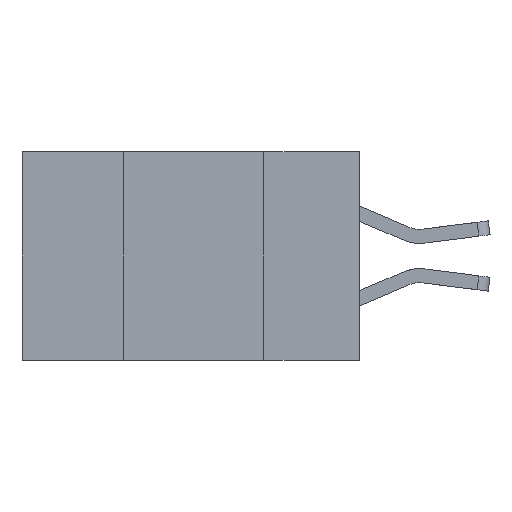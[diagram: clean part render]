
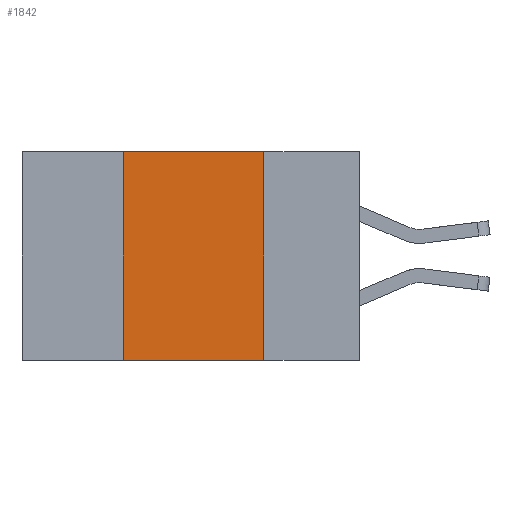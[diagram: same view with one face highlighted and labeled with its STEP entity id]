
A CAD part, left-side view. The second image highlights one B-rep face of the part: STEP entity #1842.
In plain terms, the highlighted planar face has unit normal (-1, 0, 0).
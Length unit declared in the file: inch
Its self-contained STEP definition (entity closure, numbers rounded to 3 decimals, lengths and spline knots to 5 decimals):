
#111 = FACE_OUTER_BOUND ( 'NONE', #4299, .T. ) ;
#204 = LINE ( 'NONE', #1067, #6539 ) ;
#880 = EDGE_CURVE ( 'NONE', #5905, #8308, #2870, .T. ) ;
#1003 = EDGE_CURVE ( 'NONE', #5375, #8308, #4313, .T. ) ;
#1067 = CARTESIAN_POINT ( 'NONE',  ( 0., 0.6, 0. ) ) ;
#1464 = AXIS2_PLACEMENT_3D ( 'NONE', #8762, #1615, #1802 ) ;
#1575 = VECTOR ( 'NONE', #8467, 39.37008 ) ;
#1615 = DIRECTION ( 'NONE',  ( 1., 0., 0. ) ) ;
#1802 = DIRECTION ( 'NONE',  ( 0., 0., -1. ) ) ;
#1842 = ADVANCED_FACE ( 'NONE', ( #111 ), #4460, .F. ) ;
#2870 = LINE ( 'NONE', #7503, #6959 ) ;
#2989 = CARTESIAN_POINT ( 'NONE',  ( 0., 0.42, 0. ) ) ;
#3553 = ORIENTED_EDGE ( 'NONE', *, *, #4129, .F. ) ;
#4002 = CARTESIAN_POINT ( 'NONE',  ( 0., 0.42, -0.37 ) ) ;
#4129 = EDGE_CURVE ( 'NONE', #5905, #6833, #8019, .T. ) ;
#4299 = EDGE_LOOP ( 'NONE', ( #8887, #4461, #3553, #9949 ) ) ;
#4313 = LINE ( 'NONE', #8397, #1575 ) ;
#4460 = PLANE ( 'NONE',  #1464 ) ;
#4461 = ORIENTED_EDGE ( 'NONE', *, *, #9060, .F. ) ;
#5375 = VERTEX_POINT ( 'NONE', #10539 ) ;
#5905 = VERTEX_POINT ( 'NONE', #4002 ) ;
#6155 = VECTOR ( 'NONE', #7654, 39.37008 ) ;
#6539 = VECTOR ( 'NONE', #10090, 39.37008 ) ;
#6833 = VERTEX_POINT ( 'NONE', #2989 ) ;
#6959 = VECTOR ( 'NONE', #9754, 39.37008 ) ;
#7503 = CARTESIAN_POINT ( 'NONE',  ( 0., 0.6, -0.37 ) ) ;
#7654 = DIRECTION ( 'NONE',  ( 0., 0., 1. ) ) ;
#7668 = CARTESIAN_POINT ( 'NONE',  ( 0., 0.42, 0. ) ) ;
#7683 = CARTESIAN_POINT ( 'NONE',  ( 0., 0.17, -0.37 ) ) ;
#8019 = LINE ( 'NONE', #7668, #6155 ) ;
#8308 = VERTEX_POINT ( 'NONE', #7683 ) ;
#8397 = CARTESIAN_POINT ( 'NONE',  ( 0., 0.17, 0. ) ) ;
#8467 = DIRECTION ( 'NONE',  ( 0., 0., -1. ) ) ;
#8762 = CARTESIAN_POINT ( 'NONE',  ( 0., 0.6, 0. ) ) ;
#8887 = ORIENTED_EDGE ( 'NONE', *, *, #1003, .F. ) ;
#9060 = EDGE_CURVE ( 'NONE', #6833, #5375, #204, .T. ) ;
#9754 = DIRECTION ( 'NONE',  ( 0., -1., 0. ) ) ;
#9949 = ORIENTED_EDGE ( 'NONE', *, *, #880, .T. ) ;
#10090 = DIRECTION ( 'NONE',  ( 0., -1., 0. ) ) ;
#10539 = CARTESIAN_POINT ( 'NONE',  ( 0., 0.17, 0. ) ) ;
